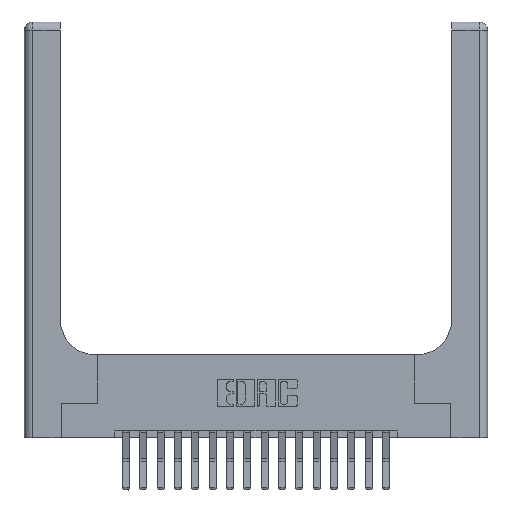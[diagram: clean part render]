
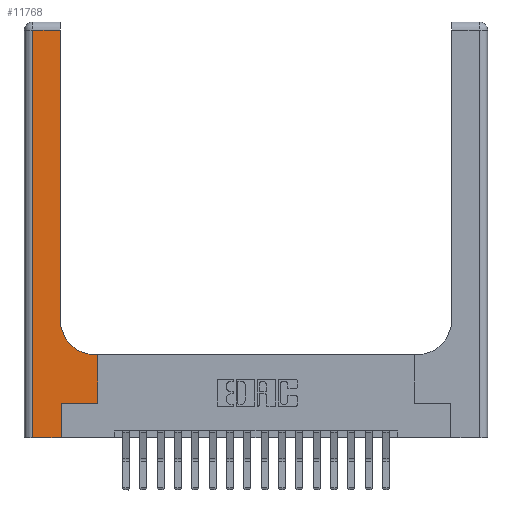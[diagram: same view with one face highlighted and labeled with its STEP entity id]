
A CAD part, top view. The second image highlights one B-rep face of the part: STEP entity #11768.
In plain terms, the highlighted planar face has unit normal (0, 0, 1).
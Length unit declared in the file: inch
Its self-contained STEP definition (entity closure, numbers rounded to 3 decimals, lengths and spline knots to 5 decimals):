
#540 = ORIENTED_EDGE ( 'NONE', *, *, #14572, .T. ) ;
#591 = EDGE_LOOP ( 'NONE', ( #3949, #15678, #540, #10904, #11423, #11742, #13164, #4040, #17048 ) ) ;
#928 = VERTEX_POINT ( 'NONE', #12980 ) ;
#1053 = CARTESIAN_POINT ( 'NONE',  ( 0.265, 0., 0.37 ) ) ;
#1062 = VECTOR ( 'NONE', #13774, 39.37008 ) ;
#1931 = AXIS2_PLACEMENT_3D ( 'NONE', #4655, #3274, #9278 ) ;
#2012 = EDGE_CURVE ( 'NONE', #928, #2871, #11057, .T. ) ;
#2105 = VERTEX_POINT ( 'NONE', #14128 ) ;
#2158 = EDGE_CURVE ( 'NONE', #4534, #928, #12746, .T. ) ;
#2717 = EDGE_CURVE ( 'NONE', #8674, #6790, #5835, .T. ) ;
#2871 = VERTEX_POINT ( 'NONE', #15682 ) ;
#3067 = LINE ( 'NONE', #7066, #3737 ) ;
#3272 = VECTOR ( 'NONE', #7363, 39.37008 ) ;
#3274 = DIRECTION ( 'NONE',  ( 0., 0., -1. ) ) ;
#3617 = LINE ( 'NONE', #5653, #6444 ) ;
#3634 = CARTESIAN_POINT ( 'NONE',  ( 0.265, 0., 0.37 ) ) ;
#3737 = VECTOR ( 'NONE', #9808, 39.37008 ) ;
#3817 = CARTESIAN_POINT ( 'NONE',  ( 0.06, 2.94, 0.37 ) ) ;
#3949 = ORIENTED_EDGE ( 'NONE', *, *, #17630, .T. ) ;
#3994 = DIRECTION ( 'NONE',  ( -1., 0., 0. ) ) ;
#4040 = ORIENTED_EDGE ( 'NONE', *, *, #2158, .T. ) ;
#4534 = VERTEX_POINT ( 'NONE', #7205 ) ;
#4655 = CARTESIAN_POINT ( 'NONE',  ( 0.51, 0.85, 0.37 ) ) ;
#5517 = LINE ( 'NONE', #14576, #14584 ) ;
#5653 = CARTESIAN_POINT ( 'NONE',  ( 0.26, 3., 0.37 ) ) ;
#5835 = LINE ( 'NONE', #14769, #3272 ) ;
#5896 = VERTEX_POINT ( 'NONE', #15240 ) ;
#6074 = CARTESIAN_POINT ( 'NONE',  ( 0., 0., 0.37 ) ) ;
#6108 = LINE ( 'NONE', #6074, #15397 ) ;
#6444 = VECTOR ( 'NONE', #17306, 39.37008 ) ;
#6790 = VERTEX_POINT ( 'NONE', #3817 ) ;
#7066 = CARTESIAN_POINT ( 'NONE',  ( 0.06, 3., 0.37 ) ) ;
#7205 = CARTESIAN_POINT ( 'NONE',  ( 0.528, 0.6, 0.37 ) ) ;
#7363 = DIRECTION ( 'NONE',  ( -1., 0., 0. ) ) ;
#7380 = DIRECTION ( 'NONE',  ( 1., 0., 0. ) ) ;
#8259 = VECTOR ( 'NONE', #9937, 39.37008 ) ;
#8279 = EDGE_CURVE ( 'NONE', #2105, #9786, #6108, .T. ) ;
#8356 = PLANE ( 'NONE',  #15513 ) ;
#8406 = VECTOR ( 'NONE', #11262, 39.37008 ) ;
#8674 = VERTEX_POINT ( 'NONE', #18649 ) ;
#8802 = DIRECTION ( 'NONE',  ( 1., 0., 0. ) ) ;
#9011 = EDGE_CURVE ( 'NONE', #5896, #4534, #9694, .T. ) ;
#9278 = DIRECTION ( 'NONE',  ( 1., 0., 0. ) ) ;
#9694 = LINE ( 'NONE', #18072, #1062 ) ;
#9786 = VERTEX_POINT ( 'NONE', #3634 ) ;
#9808 = DIRECTION ( 'NONE',  ( 0., -1., 0. ) ) ;
#9937 = DIRECTION ( 'NONE',  ( 0., 1., 0. ) ) ;
#10904 = ORIENTED_EDGE ( 'NONE', *, *, #8279, .T. ) ;
#11057 = CIRCLE ( 'NONE', #1931, 0.25 ) ;
#11071 = CARTESIAN_POINT ( 'NONE',  ( 0.26, 0.6, 0.37 ) ) ;
#11262 = DIRECTION ( 'NONE',  ( -1., 0., 0. ) ) ;
#11293 = DIRECTION ( 'NONE',  ( 0., 0., -1. ) ) ;
#11423 = ORIENTED_EDGE ( 'NONE', *, *, #18266, .T. ) ;
#11426 = CARTESIAN_POINT ( 'NONE',  ( 0., 3., 0.37 ) ) ;
#11742 = ORIENTED_EDGE ( 'NONE', *, *, #17196, .T. ) ;
#11768 = ADVANCED_FACE ( 'NONE', ( #17525 ), #8356, .F. ) ;
#12237 = LINE ( 'NONE', #1053, #8259 ) ;
#12746 = LINE ( 'NONE', #11071, #8406 ) ;
#12980 = CARTESIAN_POINT ( 'NONE',  ( 0.51, 0.6, 0.37 ) ) ;
#13164 = ORIENTED_EDGE ( 'NONE', *, *, #9011, .T. ) ;
#13774 = DIRECTION ( 'NONE',  ( 0., 1., 0. ) ) ;
#14128 = CARTESIAN_POINT ( 'NONE',  ( 0.06, 0., 0.37 ) ) ;
#14572 = EDGE_CURVE ( 'NONE', #6790, #2105, #3067, .T. ) ;
#14576 = CARTESIAN_POINT ( 'NONE',  ( 0.265, 0.25, 0.37 ) ) ;
#14584 = VECTOR ( 'NONE', #8802, 39.37008 ) ;
#14769 = CARTESIAN_POINT ( 'NONE',  ( 0., 2.94, 0.37 ) ) ;
#15240 = CARTESIAN_POINT ( 'NONE',  ( 0.528, 0.25, 0.37 ) ) ;
#15397 = VECTOR ( 'NONE', #7380, 39.37008 ) ;
#15513 = AXIS2_PLACEMENT_3D ( 'NONE', #11426, #11293, #3994 ) ;
#15678 = ORIENTED_EDGE ( 'NONE', *, *, #2717, .T. ) ;
#15682 = CARTESIAN_POINT ( 'NONE',  ( 0.26, 0.85, 0.37 ) ) ;
#16869 = VERTEX_POINT ( 'NONE', #18227 ) ;
#17048 = ORIENTED_EDGE ( 'NONE', *, *, #2012, .T. ) ;
#17196 = EDGE_CURVE ( 'NONE', #16869, #5896, #5517, .T. ) ;
#17306 = DIRECTION ( 'NONE',  ( 0., 1., 0. ) ) ;
#17525 = FACE_OUTER_BOUND ( 'NONE', #591, .T. ) ;
#17630 = EDGE_CURVE ( 'NONE', #2871, #8674, #3617, .T. ) ;
#18072 = CARTESIAN_POINT ( 'NONE',  ( 0.528, 0.25, 0.37 ) ) ;
#18227 = CARTESIAN_POINT ( 'NONE',  ( 0.265, 0.25, 0.37 ) ) ;
#18266 = EDGE_CURVE ( 'NONE', #9786, #16869, #12237, .T. ) ;
#18649 = CARTESIAN_POINT ( 'NONE',  ( 0.26, 2.94, 0.37 ) ) ;
